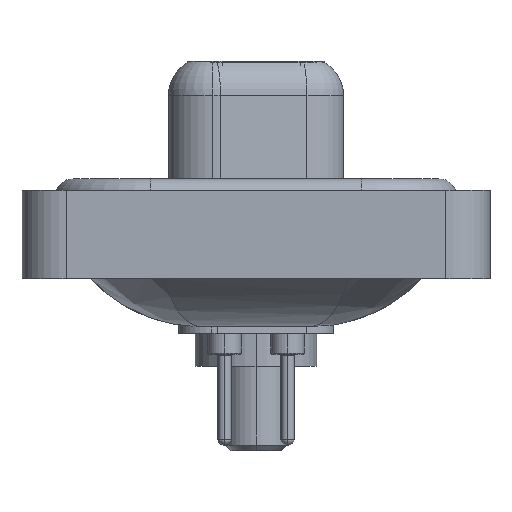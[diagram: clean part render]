
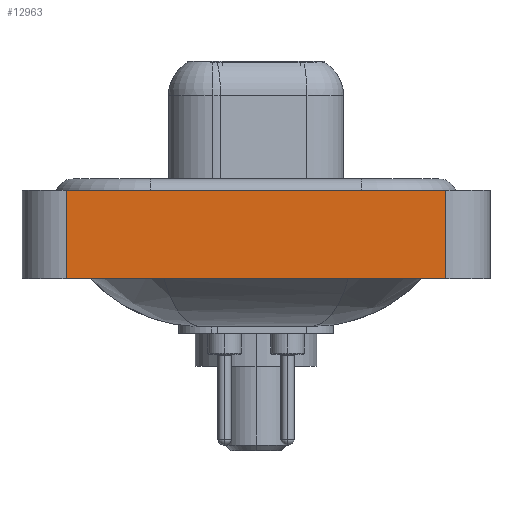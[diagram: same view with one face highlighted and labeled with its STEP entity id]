
A CAD part, left-side view. The second image highlights one B-rep face of the part: STEP entity #12963.
In plain terms, the highlighted planar face has unit normal (-1, 0, 0).
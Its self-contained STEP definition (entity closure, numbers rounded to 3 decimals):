
#613 = FACE_OUTER_BOUND ( 'NONE', #1087, .T. ) ;
#701 = VERTEX_POINT ( 'NONE', #2664 ) ;
#1087 = EDGE_LOOP ( 'NONE', ( #6713, #10272, #18770, #16567 ) ) ;
#1916 = DIRECTION ( 'NONE',  ( 0., 0., 1. ) ) ;
#2242 = DIRECTION ( 'NONE',  ( -1., 0., 0. ) ) ;
#2664 = CARTESIAN_POINT ( 'NONE',  ( -7.25, -8.55, 0.4 ) ) ;
#2780 = VECTOR ( 'NONE', #4347, 1000. ) ;
#2885 = VECTOR ( 'NONE', #17140, 1000. ) ;
#3626 = CARTESIAN_POINT ( 'NONE',  ( -7.25, 8.55, -3.6 ) ) ;
#3962 = CARTESIAN_POINT ( 'NONE',  ( -7.25, 8.55, 0.4 ) ) ;
#4067 = CARTESIAN_POINT ( 'NONE',  ( -7.25, -8.55, -3.6 ) ) ;
#4242 = EDGE_CURVE ( 'NONE', #17052, #701, #4801, .T. ) ;
#4347 = DIRECTION ( 'NONE',  ( 0., 0., 1. ) ) ;
#4383 = DIRECTION ( 'NONE',  ( 0., -1., 0. ) ) ;
#4801 = LINE ( 'NONE', #18881, #2885 ) ;
#6713 = ORIENTED_EDGE ( 'NONE', *, *, #8304, .T. ) ;
#7470 = VERTEX_POINT ( 'NONE', #16267 ) ;
#7916 = VERTEX_POINT ( 'NONE', #9907 ) ;
#8304 = EDGE_CURVE ( 'NONE', #7916, #701, #8558, .T. ) ;
#8558 = LINE ( 'NONE', #4067, #2780 ) ;
#8618 = PLANE ( 'NONE',  #15439 ) ;
#8678 = VECTOR ( 'NONE', #4383, 1000. ) ;
#9249 = EDGE_CURVE ( 'NONE', #7470, #17052, #18686, .T. ) ;
#9728 = CARTESIAN_POINT ( 'NONE',  ( -7.25, -8.55, -3.6 ) ) ;
#9907 = CARTESIAN_POINT ( 'NONE',  ( -7.25, -8.55, -3.6 ) ) ;
#10272 = ORIENTED_EDGE ( 'NONE', *, *, #4242, .F. ) ;
#11097 = VECTOR ( 'NONE', #1916, 1000. ) ;
#11967 = LINE ( 'NONE', #18141, #8678 ) ;
#12681 = EDGE_CURVE ( 'NONE', #7470, #7916, #11967, .T. ) ;
#12963 = ADVANCED_FACE ( 'NONE', ( #613 ), #8618, .T. ) ;
#15439 = AXIS2_PLACEMENT_3D ( 'NONE', #9728, #2242, #15869 ) ;
#15869 = DIRECTION ( 'NONE',  ( 0., 0., 1. ) ) ;
#16267 = CARTESIAN_POINT ( 'NONE',  ( -7.25, 8.55, -3.6 ) ) ;
#16567 = ORIENTED_EDGE ( 'NONE', *, *, #12681, .T. ) ;
#17052 = VERTEX_POINT ( 'NONE', #3962 ) ;
#17140 = DIRECTION ( 'NONE',  ( 0., -1., 0. ) ) ;
#18141 = CARTESIAN_POINT ( 'NONE',  ( -7.25, -8.55, -3.6 ) ) ;
#18686 = LINE ( 'NONE', #3626, #11097 ) ;
#18770 = ORIENTED_EDGE ( 'NONE', *, *, #9249, .F. ) ;
#18881 = CARTESIAN_POINT ( 'NONE',  ( -7.25, -8.55, 0.4 ) ) ;
